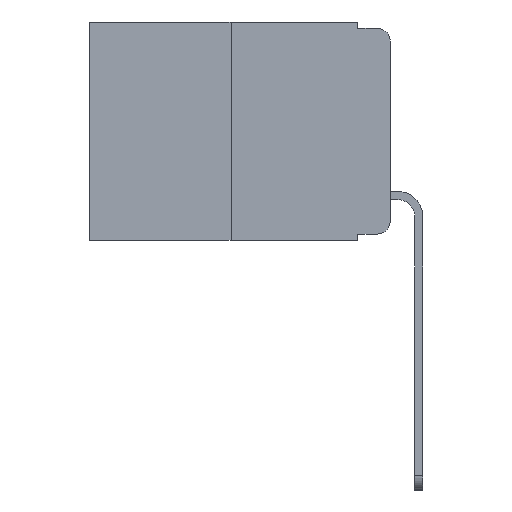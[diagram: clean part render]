
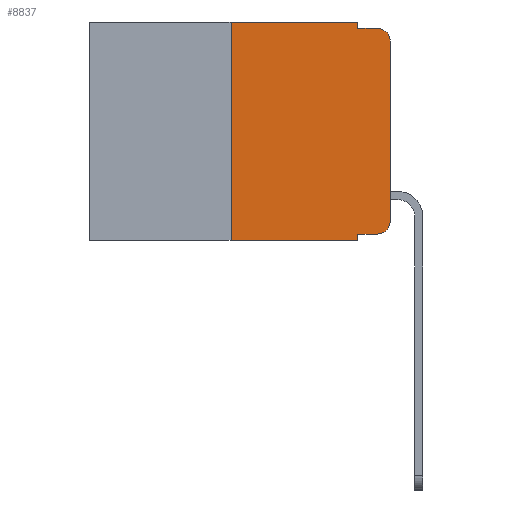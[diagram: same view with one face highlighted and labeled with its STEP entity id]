
A CAD part, left-side view. The second image highlights one B-rep face of the part: STEP entity #8837.
In plain terms, the highlighted planar face has unit normal (-1, 0, 0).
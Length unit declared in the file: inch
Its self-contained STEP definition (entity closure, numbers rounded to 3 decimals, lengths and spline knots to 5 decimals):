
#176 = CARTESIAN_POINT ( 'NONE',  ( 0., 0.25, 0. ) ) ;
#178 = CARTESIAN_POINT ( 'NONE',  ( 0., 0.02, -0.01 ) ) ;
#434 = LINE ( 'NONE', #9636, #11153 ) ;
#710 = FACE_OUTER_BOUND ( 'NONE', #9295, .T. ) ;
#1198 = VERTEX_POINT ( 'NONE', #4316 ) ;
#1210 = PLANE ( 'NONE',  #2216 ) ;
#1789 = ORIENTED_EDGE ( 'NONE', *, *, #4266, .F. ) ;
#1820 = EDGE_CURVE ( 'NONE', #7716, #2859, #10532, .T. ) ;
#1958 = DIRECTION ( 'NONE',  ( 0., -1., 0. ) ) ;
#1995 = VERTEX_POINT ( 'NONE', #12766 ) ;
#2160 = DIRECTION ( 'NONE',  ( 0., 0., 1. ) ) ;
#2216 = AXIS2_PLACEMENT_3D ( 'NONE', #4956, #13633, #2379 ) ;
#2379 = DIRECTION ( 'NONE',  ( 0., 0., -1. ) ) ;
#2453 = CARTESIAN_POINT ( 'NONE',  ( 0., 0.051, -0.343 ) ) ;
#2457 = ORIENTED_EDGE ( 'NONE', *, *, #4152, .T. ) ;
#2822 = LINE ( 'NONE', #13505, #13429 ) ;
#2859 = VERTEX_POINT ( 'NONE', #2453 ) ;
#2903 = VERTEX_POINT ( 'NONE', #176 ) ;
#3084 = DIRECTION ( 'NONE',  ( -1., 0., 0. ) ) ;
#3122 = CARTESIAN_POINT ( 'NONE',  ( 0., 0.051, -0.01 ) ) ;
#3180 = DIRECTION ( 'NONE',  ( 0., 0., -1. ) ) ;
#3278 = ORIENTED_EDGE ( 'NONE', *, *, #4044, .T. ) ;
#3760 = CARTESIAN_POINT ( 'NONE',  ( 0., 0., -0.313 ) ) ;
#3885 = VECTOR ( 'NONE', #3180, 39.37008 ) ;
#4034 = VERTEX_POINT ( 'NONE', #3760 ) ;
#4044 = EDGE_CURVE ( 'NONE', #4034, #10695, #11880, .T. ) ;
#4152 = EDGE_CURVE ( 'NONE', #10695, #12503, #7711, .T. ) ;
#4174 = EDGE_CURVE ( 'NONE', #1198, #12503, #13289, .T. ) ;
#4200 = EDGE_CURVE ( 'NONE', #10332, #1198, #4275, .T. ) ;
#4244 = EDGE_CURVE ( 'NONE', #7716, #2903, #434, .T. ) ;
#4266 = EDGE_CURVE ( 'NONE', #11448, #2859, #2822, .T. ) ;
#4275 = LINE ( 'NONE', #10510, #3885 ) ;
#4316 = CARTESIAN_POINT ( 'NONE',  ( 0., 0.051, -0.01 ) ) ;
#4336 = EDGE_CURVE ( 'NONE', #11448, #1995, #5093, .T. ) ;
#4352 = EDGE_CURVE ( 'NONE', #1995, #4034, #7873, .T. ) ;
#4558 = CARTESIAN_POINT ( 'NONE',  ( 0., 0.051, -0.333 ) ) ;
#4913 = ORIENTED_EDGE ( 'NONE', *, *, #12164, .F. ) ;
#4956 = CARTESIAN_POINT ( 'NONE',  ( 0., 0.473, 0. ) ) ;
#5026 = AXIS2_PLACEMENT_3D ( 'NONE', #12697, #6691, #8589 ) ;
#5093 = LINE ( 'NONE', #4558, #10563 ) ;
#5506 = AXIS2_PLACEMENT_3D ( 'NONE', #9446, #3084, #10436 ) ;
#5621 = DIRECTION ( 'NONE',  ( 0., -1., 0. ) ) ;
#5810 = ORIENTED_EDGE ( 'NONE', *, *, #4244, .F. ) ;
#5989 = CARTESIAN_POINT ( 'NONE',  ( 0., 0., 0. ) ) ;
#6295 = DIRECTION ( 'NONE',  ( 0., -1., 0. ) ) ;
#6560 = VECTOR ( 'NONE', #11965, 39.37008 ) ;
#6691 = DIRECTION ( 'NONE',  ( -1., 0., 0. ) ) ;
#7487 = VECTOR ( 'NONE', #11726, 39.37008 ) ;
#7546 = CARTESIAN_POINT ( 'NONE',  ( 0., 0.473, -0.343 ) ) ;
#7711 = CIRCLE ( 'NONE', #5506, 0.02 ) ;
#7716 = VERTEX_POINT ( 'NONE', #9120 ) ;
#7873 = CIRCLE ( 'NONE', #5026, 0.02 ) ;
#8064 = ORIENTED_EDGE ( 'NONE', *, *, #4352, .T. ) ;
#8230 = VECTOR ( 'NONE', #6295, 39.37008 ) ;
#8589 = DIRECTION ( 'NONE',  ( 0., 0., -1. ) ) ;
#8662 = ORIENTED_EDGE ( 'NONE', *, *, #4200, .F. ) ;
#8697 = CARTESIAN_POINT ( 'NONE',  ( 0., 0., -0.03 ) ) ;
#8837 = ADVANCED_FACE ( 'NONE', ( #710 ), #1210, .F. ) ;
#9120 = CARTESIAN_POINT ( 'NONE',  ( 0., 0.25, -0.343 ) ) ;
#9295 = EDGE_LOOP ( 'NONE', ( #3278, #2457, #13112, #8662, #4913, #5810, #12827, #1789, #9361, #8064 ) ) ;
#9361 = ORIENTED_EDGE ( 'NONE', *, *, #4336, .T. ) ;
#9446 = CARTESIAN_POINT ( 'NONE',  ( 0., 0.02, -0.03 ) ) ;
#9636 = CARTESIAN_POINT ( 'NONE',  ( 0., 0.25, 0. ) ) ;
#10099 = VECTOR ( 'NONE', #1958, 39.37008 ) ;
#10232 = CARTESIAN_POINT ( 'NONE',  ( 0., 0.051, 0. ) ) ;
#10332 = VERTEX_POINT ( 'NONE', #10232 ) ;
#10436 = DIRECTION ( 'NONE',  ( 0., 0., -1. ) ) ;
#10510 = CARTESIAN_POINT ( 'NONE',  ( 0., 0.051, 0. ) ) ;
#10532 = LINE ( 'NONE', #7546, #7487 ) ;
#10563 = VECTOR ( 'NONE', #5621, 39.37008 ) ;
#10695 = VERTEX_POINT ( 'NONE', #8697 ) ;
#11153 = VECTOR ( 'NONE', #2160, 39.37008 ) ;
#11328 = CARTESIAN_POINT ( 'NONE',  ( 0., 0.473, 0. ) ) ;
#11448 = VERTEX_POINT ( 'NONE', #12393 ) ;
#11726 = DIRECTION ( 'NONE',  ( 0., -1., 0. ) ) ;
#11880 = LINE ( 'NONE', #5989, #6560 ) ;
#11965 = DIRECTION ( 'NONE',  ( 0., 0., 1. ) ) ;
#12164 = EDGE_CURVE ( 'NONE', #2903, #10332, #13440, .T. ) ;
#12393 = CARTESIAN_POINT ( 'NONE',  ( 0., 0.051, -0.333 ) ) ;
#12503 = VERTEX_POINT ( 'NONE', #178 ) ;
#12571 = DIRECTION ( 'NONE',  ( 0., 0., -1. ) ) ;
#12697 = CARTESIAN_POINT ( 'NONE',  ( 0., 0.02, -0.313 ) ) ;
#12766 = CARTESIAN_POINT ( 'NONE',  ( 0., 0.02, -0.333 ) ) ;
#12827 = ORIENTED_EDGE ( 'NONE', *, *, #1820, .T. ) ;
#13112 = ORIENTED_EDGE ( 'NONE', *, *, #4174, .F. ) ;
#13289 = LINE ( 'NONE', #3122, #10099 ) ;
#13429 = VECTOR ( 'NONE', #12571, 39.37008 ) ;
#13440 = LINE ( 'NONE', #11328, #8230 ) ;
#13505 = CARTESIAN_POINT ( 'NONE',  ( 0., 0.051, 0. ) ) ;
#13633 = DIRECTION ( 'NONE',  ( 1., 0., 0. ) ) ;
